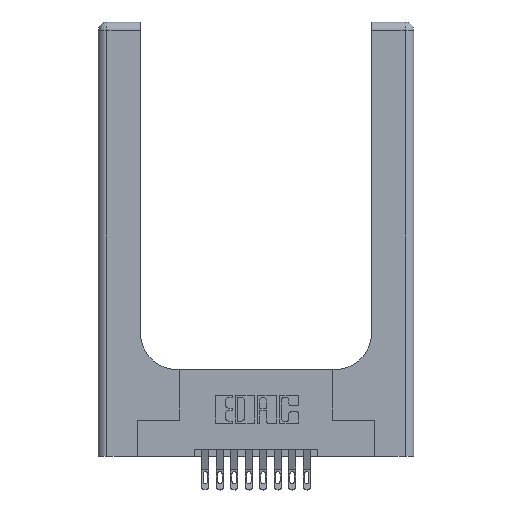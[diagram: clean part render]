
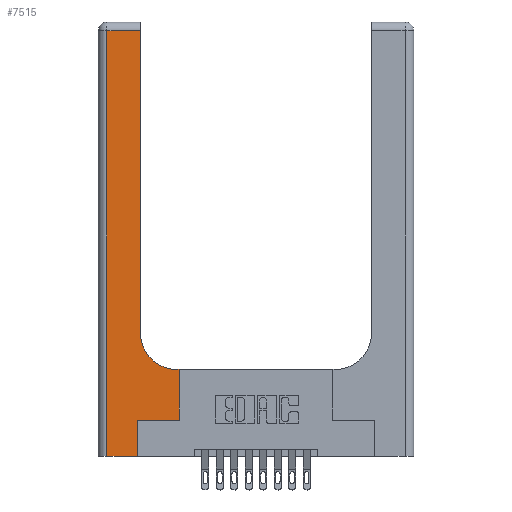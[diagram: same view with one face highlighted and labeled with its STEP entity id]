
A CAD part, top view. The second image highlights one B-rep face of the part: STEP entity #7515.
In plain terms, the highlighted planar face has unit normal (0, 0, 1).
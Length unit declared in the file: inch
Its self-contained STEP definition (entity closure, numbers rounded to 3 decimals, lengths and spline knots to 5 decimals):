
#116 = CARTESIAN_POINT ( 'NONE',  ( 0.2915, 3., 0.37 ) ) ;
#643 = LINE ( 'NONE', #2381, #13311 ) ;
#656 = VECTOR ( 'NONE', #12098, 39.37008 ) ;
#705 = FACE_OUTER_BOUND ( 'NONE', #13345, .T. ) ;
#895 = VERTEX_POINT ( 'NONE', #14813 ) ;
#1134 = CARTESIAN_POINT ( 'NONE',  ( 0.5585, 0.25, 0.37 ) ) ;
#1347 = CIRCLE ( 'NONE', #13035, 0.25 ) ;
#1471 = ORIENTED_EDGE ( 'NONE', *, *, #15605, .T. ) ;
#1992 = VECTOR ( 'NONE', #15373, 39.37008 ) ;
#2271 = ORIENTED_EDGE ( 'NONE', *, *, #2713, .T. ) ;
#2367 = LINE ( 'NONE', #13865, #11313 ) ;
#2381 = CARTESIAN_POINT ( 'NONE',  ( 0.269, 0., 0.37 ) ) ;
#2713 = EDGE_CURVE ( 'NONE', #14513, #14400, #12126, .T. ) ;
#2751 = DIRECTION ( 'NONE',  ( 0., 0., -1. ) ) ;
#3339 = DIRECTION ( 'NONE',  ( 1., 0., 0. ) ) ;
#3355 = EDGE_CURVE ( 'NONE', #10195, #13535, #10549, .T. ) ;
#3472 = ORIENTED_EDGE ( 'NONE', *, *, #9559, .T. ) ;
#3625 = CARTESIAN_POINT ( 'NONE',  ( 0.2915, 0.85, 0.37 ) ) ;
#3689 = VECTOR ( 'NONE', #12798, 39.37008 ) ;
#3745 = EDGE_CURVE ( 'NONE', #895, #4770, #2367, .T. ) ;
#3868 = ORIENTED_EDGE ( 'NONE', *, *, #9353, .T. ) ;
#4082 = LINE ( 'NONE', #116, #3689 ) ;
#4169 = CARTESIAN_POINT ( 'NONE',  ( 0., 3., 0.37 ) ) ;
#4254 = VERTEX_POINT ( 'NONE', #9806 ) ;
#4372 = AXIS2_PLACEMENT_3D ( 'NONE', #4169, #14308, #6715 ) ;
#4543 = CARTESIAN_POINT ( 'NONE',  ( 0.269, 0.25, 0.37 ) ) ;
#4770 = VERTEX_POINT ( 'NONE', #12247 ) ;
#5174 = CARTESIAN_POINT ( 'NONE',  ( 0.5585, 0.25, 0.37 ) ) ;
#5697 = CARTESIAN_POINT ( 'NONE',  ( 0.06, 3., 0.37 ) ) ;
#6021 = ORIENTED_EDGE ( 'NONE', *, *, #11555, .T. ) ;
#6438 = ORIENTED_EDGE ( 'NONE', *, *, #3745, .T. ) ;
#6656 = CARTESIAN_POINT ( 'NONE',  ( 0.5415, 0.6, 0.37 ) ) ;
#6715 = DIRECTION ( 'NONE',  ( -1., 0., 0. ) ) ;
#6725 = LINE ( 'NONE', #5697, #656 ) ;
#6900 = DIRECTION ( 'NONE',  ( -1., 0., 0. ) ) ;
#7059 = EDGE_CURVE ( 'NONE', #13535, #9204, #10840, .T. ) ;
#7515 = ADVANCED_FACE ( 'NONE', ( #705 ), #13046, .F. ) ;
#7856 = CARTESIAN_POINT ( 'NONE',  ( 0.06, 2.94, 0.37 ) ) ;
#9204 = VERTEX_POINT ( 'NONE', #6656 ) ;
#9353 = EDGE_CURVE ( 'NONE', #4254, #10195, #9791, .T. ) ;
#9559 = EDGE_CURVE ( 'NONE', #4770, #4254, #643, .T. ) ;
#9791 = LINE ( 'NONE', #4543, #12723 ) ;
#9806 = CARTESIAN_POINT ( 'NONE',  ( 0.269, 0.25, 0.37 ) ) ;
#10012 = DIRECTION ( 'NONE',  ( 0., 1., 0. ) ) ;
#10195 = VERTEX_POINT ( 'NONE', #1134 ) ;
#10390 = CARTESIAN_POINT ( 'NONE',  ( 0.5415, 0.85, 0.37 ) ) ;
#10459 = VECTOR ( 'NONE', #6900, 39.37008 ) ;
#10549 = LINE ( 'NONE', #5174, #13471 ) ;
#10640 = ORIENTED_EDGE ( 'NONE', *, *, #3355, .T. ) ;
#10840 = LINE ( 'NONE', #13219, #10459 ) ;
#11035 = ORIENTED_EDGE ( 'NONE', *, *, #7059, .T. ) ;
#11313 = VECTOR ( 'NONE', #12609, 39.37008 ) ;
#11555 = EDGE_CURVE ( 'NONE', #14400, #895, #6725, .T. ) ;
#11642 = DIRECTION ( 'NONE',  ( 1., 0., 0. ) ) ;
#12098 = DIRECTION ( 'NONE',  ( 0., -1., 0. ) ) ;
#12126 = LINE ( 'NONE', #15351, #1992 ) ;
#12247 = CARTESIAN_POINT ( 'NONE',  ( 0.269, 0., 0.37 ) ) ;
#12609 = DIRECTION ( 'NONE',  ( 1., 0., 0. ) ) ;
#12723 = VECTOR ( 'NONE', #3339, 39.37008 ) ;
#12779 = VERTEX_POINT ( 'NONE', #3625 ) ;
#12798 = DIRECTION ( 'NONE',  ( 0., 1., 0. ) ) ;
#13035 = AXIS2_PLACEMENT_3D ( 'NONE', #10390, #2751, #11642 ) ;
#13046 = PLANE ( 'NONE',  #4372 ) ;
#13067 = CARTESIAN_POINT ( 'NONE',  ( 0.2915, 2.94, 0.37 ) ) ;
#13219 = CARTESIAN_POINT ( 'NONE',  ( 0.2915, 0.6, 0.37 ) ) ;
#13311 = VECTOR ( 'NONE', #10012, 39.37008 ) ;
#13345 = EDGE_LOOP ( 'NONE', ( #1471, #2271, #6021, #6438, #3472, #3868, #10640, #11035, #14753 ) ) ;
#13471 = VECTOR ( 'NONE', #14050, 39.37008 ) ;
#13535 = VERTEX_POINT ( 'NONE', #15314 ) ;
#13865 = CARTESIAN_POINT ( 'NONE',  ( 0., 0., 0.37 ) ) ;
#14050 = DIRECTION ( 'NONE',  ( 0., 1., 0. ) ) ;
#14308 = DIRECTION ( 'NONE',  ( 0., 0., -1. ) ) ;
#14385 = EDGE_CURVE ( 'NONE', #9204, #12779, #1347, .T. ) ;
#14400 = VERTEX_POINT ( 'NONE', #7856 ) ;
#14513 = VERTEX_POINT ( 'NONE', #13067 ) ;
#14753 = ORIENTED_EDGE ( 'NONE', *, *, #14385, .T. ) ;
#14813 = CARTESIAN_POINT ( 'NONE',  ( 0.06, 0., 0.37 ) ) ;
#15314 = CARTESIAN_POINT ( 'NONE',  ( 0.5585, 0.6, 0.37 ) ) ;
#15351 = CARTESIAN_POINT ( 'NONE',  ( 0., 2.94, 0.37 ) ) ;
#15373 = DIRECTION ( 'NONE',  ( -1., 0., 0. ) ) ;
#15605 = EDGE_CURVE ( 'NONE', #12779, #14513, #4082, .T. ) ;
